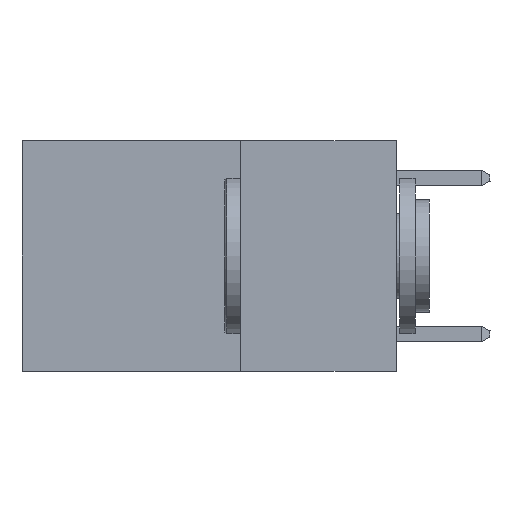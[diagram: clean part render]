
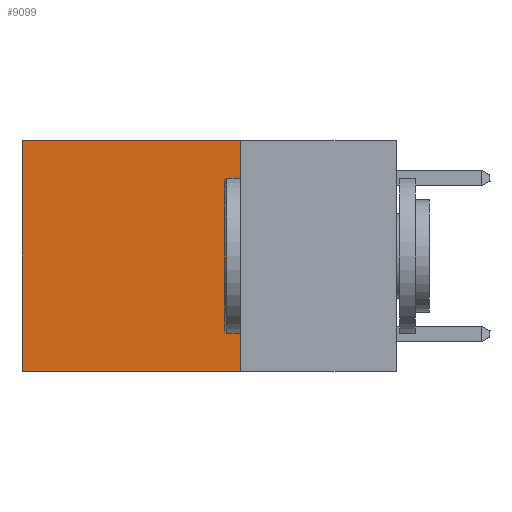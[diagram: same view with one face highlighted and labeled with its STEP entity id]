
A CAD part, left-side view. The second image highlights one B-rep face of the part: STEP entity #9099.
In plain terms, the highlighted planar face has unit normal (-1, 0, 0).
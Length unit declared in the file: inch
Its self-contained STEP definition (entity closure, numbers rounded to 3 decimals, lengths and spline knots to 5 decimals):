
#1669 = LINE ( 'NONE', #6277, #24740 ) ;
#1702 = VECTOR ( 'NONE', #20106, 39.37008 ) ;
#1865 = EDGE_CURVE ( 'NONE', #27433, #2814, #2157, .T. ) ;
#1944 = CARTESIAN_POINT ( 'NONE',  ( 0.2625, 0.6, 0. ) ) ;
#2157 = LINE ( 'NONE', #11172, #1702 ) ;
#2199 = VERTEX_POINT ( 'NONE', #23991 ) ;
#2814 = VERTEX_POINT ( 'NONE', #1944 ) ;
#3366 = DIRECTION ( 'NONE',  ( 0., 0., -1. ) ) ;
#3919 = ORIENTED_EDGE ( 'NONE', *, *, #8784, .F. ) ;
#4732 = EDGE_LOOP ( 'NONE', ( #23327, #19709, #3919, #23780 ) ) ;
#5806 = LINE ( 'NONE', #27961, #11864 ) ;
#6277 = CARTESIAN_POINT ( 'NONE',  ( 0.2625, 0.6, 0. ) ) ;
#7334 = CARTESIAN_POINT ( 'NONE',  ( 0.2625, 0.25, 0. ) ) ;
#8085 = FACE_OUTER_BOUND ( 'NONE', #4732, .T. ) ;
#8784 = EDGE_CURVE ( 'NONE', #27433, #2199, #25499, .T. ) ;
#9099 = ADVANCED_FACE ( 'NONE', ( #8085 ), #23750, .F. ) ;
#10024 = CARTESIAN_POINT ( 'NONE',  ( 0.2625, 0.25, 0. ) ) ;
#11172 = CARTESIAN_POINT ( 'NONE',  ( 0.2625, 0.25, 0. ) ) ;
#11853 = DIRECTION ( 'NONE',  ( 0., 0., -1. ) ) ;
#11864 = VECTOR ( 'NONE', #16835, 39.37008 ) ;
#13203 = VECTOR ( 'NONE', #11853, 39.37008 ) ;
#14417 = DIRECTION ( 'NONE',  ( 1., 0., 0. ) ) ;
#16557 = CARTESIAN_POINT ( 'NONE',  ( 0.2625, 0.25, 0. ) ) ;
#16835 = DIRECTION ( 'NONE',  ( 0., 1., 0. ) ) ;
#17068 = EDGE_CURVE ( 'NONE', #2814, #18213, #1669, .T. ) ;
#18213 = VERTEX_POINT ( 'NONE', #22173 ) ;
#19709 = ORIENTED_EDGE ( 'NONE', *, *, #26682, .F. ) ;
#20106 = DIRECTION ( 'NONE',  ( 0., 1., 0. ) ) ;
#22173 = CARTESIAN_POINT ( 'NONE',  ( 0.2625, 0.6, -0.37 ) ) ;
#23117 = AXIS2_PLACEMENT_3D ( 'NONE', #10024, #14417, #3366 ) ;
#23327 = ORIENTED_EDGE ( 'NONE', *, *, #17068, .T. ) ;
#23750 = PLANE ( 'NONE',  #23117 ) ;
#23780 = ORIENTED_EDGE ( 'NONE', *, *, #1865, .T. ) ;
#23984 = DIRECTION ( 'NONE',  ( 0., 0., -1. ) ) ;
#23991 = CARTESIAN_POINT ( 'NONE',  ( 0.2625, 0.25, -0.37 ) ) ;
#24740 = VECTOR ( 'NONE', #23984, 39.37008 ) ;
#25499 = LINE ( 'NONE', #16557, #13203 ) ;
#26682 = EDGE_CURVE ( 'NONE', #2199, #18213, #5806, .T. ) ;
#27433 = VERTEX_POINT ( 'NONE', #7334 ) ;
#27961 = CARTESIAN_POINT ( 'NONE',  ( 0.2625, 0.25, -0.37 ) ) ;
